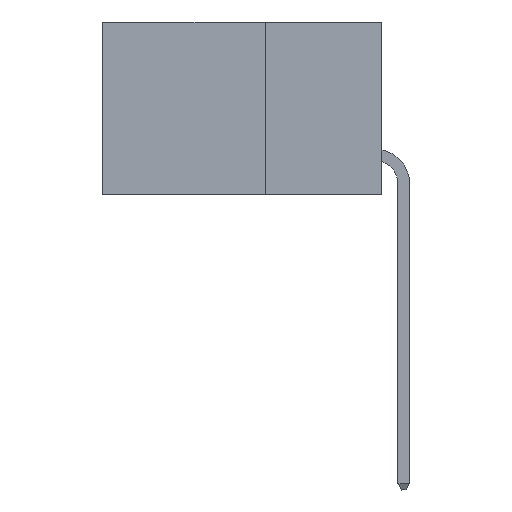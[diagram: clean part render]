
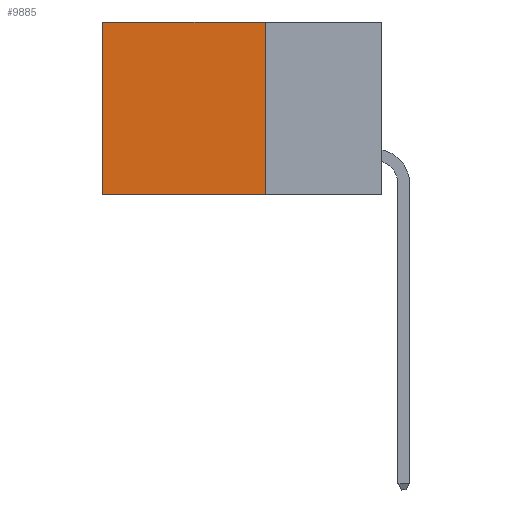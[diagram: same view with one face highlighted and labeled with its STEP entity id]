
A CAD part, left-side view. The second image highlights one B-rep face of the part: STEP entity #9885.
In plain terms, the highlighted planar face has unit normal (-1, 0, 0).
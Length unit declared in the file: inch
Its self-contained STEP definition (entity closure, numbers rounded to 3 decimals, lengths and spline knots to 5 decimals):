
#990 = CARTESIAN_POINT ( 'NONE',  ( 0.2875, 0.6, 0. ) ) ;
#1910 = EDGE_CURVE ( 'NONE', #22159, #14978, #33548, .T. ) ;
#2730 = EDGE_CURVE ( 'NONE', #6985, #40253, #36245, .T. ) ;
#3561 = ORIENTED_EDGE ( 'NONE', *, *, #5854, .F. ) ;
#4300 = CARTESIAN_POINT ( 'NONE',  ( 0.2875, 0.25, -0.37 ) ) ;
#5070 = DIRECTION ( 'NONE',  ( 0., 0., -1. ) ) ;
#5820 = AXIS2_PLACEMENT_3D ( 'NONE', #9067, #33574, #5070 ) ;
#5854 = EDGE_CURVE ( 'NONE', #22159, #6985, #15061, .T. ) ;
#6099 = CARTESIAN_POINT ( 'NONE',  ( 0.2875, 0.25, 0. ) ) ;
#6985 = VERTEX_POINT ( 'NONE', #36568 ) ;
#9067 = CARTESIAN_POINT ( 'NONE',  ( 0.2875, 0.25, 0. ) ) ;
#9885 = ADVANCED_FACE ( 'NONE', ( #28405 ), #12186, .F. ) ;
#10428 = EDGE_CURVE ( 'NONE', #14978, #40253, #31642, .T. ) ;
#12186 = PLANE ( 'NONE',  #5820 ) ;
#13381 = VECTOR ( 'NONE', #29857, 39.37008 ) ;
#14978 = VERTEX_POINT ( 'NONE', #23055 ) ;
#15061 = LINE ( 'NONE', #33584, #13381 ) ;
#17904 = ORIENTED_EDGE ( 'NONE', *, *, #10428, .T. ) ;
#20269 = VECTOR ( 'NONE', #34945, 39.37008 ) ;
#22159 = VERTEX_POINT ( 'NONE', #6099 ) ;
#23055 = CARTESIAN_POINT ( 'NONE',  ( 0.2875, 0.6, 0. ) ) ;
#24383 = ORIENTED_EDGE ( 'NONE', *, *, #1910, .T. ) ;
#27803 = CARTESIAN_POINT ( 'NONE',  ( 0.2875, 0.25, 0. ) ) ;
#28405 = FACE_OUTER_BOUND ( 'NONE', #34103, .T. ) ;
#28558 = CARTESIAN_POINT ( 'NONE',  ( 0.2875, 0.6, -0.37 ) ) ;
#29857 = DIRECTION ( 'NONE',  ( 0., 0., -1. ) ) ;
#30535 = VECTOR ( 'NONE', #32029, 39.37008 ) ;
#31642 = LINE ( 'NONE', #990, #30535 ) ;
#31941 = ORIENTED_EDGE ( 'NONE', *, *, #2730, .F. ) ;
#32029 = DIRECTION ( 'NONE',  ( 0., 0., -1. ) ) ;
#33548 = LINE ( 'NONE', #27803, #20269 ) ;
#33574 = DIRECTION ( 'NONE',  ( 1., 0., 0. ) ) ;
#33584 = CARTESIAN_POINT ( 'NONE',  ( 0.2875, 0.25, 0. ) ) ;
#34103 = EDGE_LOOP ( 'NONE', ( #17904, #31941, #3561, #24383 ) ) ;
#34945 = DIRECTION ( 'NONE',  ( 0., 1., 0. ) ) ;
#36245 = LINE ( 'NONE', #4300, #37869 ) ;
#36568 = CARTESIAN_POINT ( 'NONE',  ( 0.2875, 0.25, -0.37 ) ) ;
#37869 = VECTOR ( 'NONE', #40671, 39.37008 ) ;
#40253 = VERTEX_POINT ( 'NONE', #28558 ) ;
#40671 = DIRECTION ( 'NONE',  ( 0., 1., 0. ) ) ;
